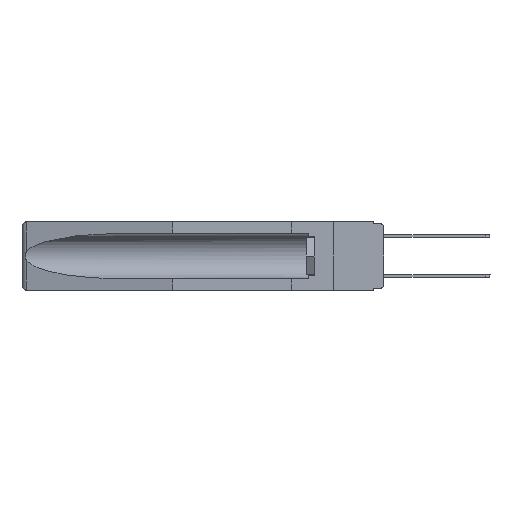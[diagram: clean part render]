
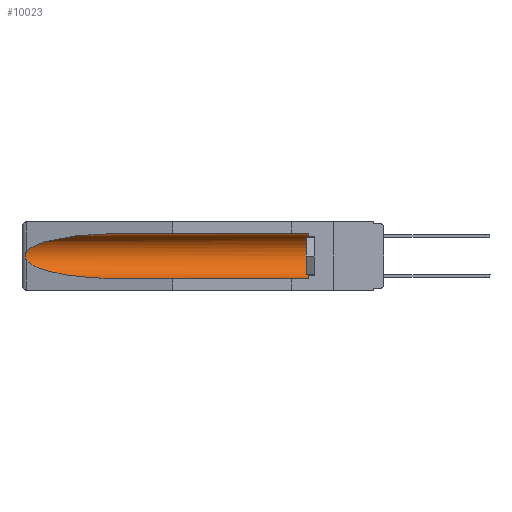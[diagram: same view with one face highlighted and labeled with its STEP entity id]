
A CAD part, left-side view. The second image highlights one B-rep face of the part: STEP entity #10023.
In plain terms, the highlighted cylindrical face has radius 2.857 mm (diameter 5.715 mm), a partial arc.
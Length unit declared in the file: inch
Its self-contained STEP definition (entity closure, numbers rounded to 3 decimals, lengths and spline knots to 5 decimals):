
#1338 = VERTEX_POINT ( 'NONE', #23030 ) ;
#1731 = CARTESIAN_POINT ( 'NONE',  ( 0.2675, 1.53308, -0.17534 ) ) ;
#1840 = CIRCLE ( 'NONE', #11067, 0.1125 ) ;
#2005 = EDGE_CURVE ( 'NONE', #6008, #21477, #17232, .T. ) ;
#2086 = CARTESIAN_POINT ( 'NONE',  ( 0.26537, 1.52718, -0.19328 ) ) ;
#2206 = CARTESIAN_POINT ( 'NONE',  ( 0.26537, 1.52718, -0.14972 ) ) ;
#2454 = EDGE_CURVE ( 'NONE', #6008, #16676, #1840, .T. ) ;
#2832 = CARTESIAN_POINT ( 'NONE',  ( 0.26537, 1.52718, -0.19328 ) ) ;
#2895 = CYLINDRICAL_SURFACE ( 'NONE', #17356, 0.1125 ) ;
#3314 = CARTESIAN_POINT ( 'NONE',  ( 0.21114, 1.30732, -0.059 ) ) ;
#3514 = EDGE_CURVE ( 'NONE', #6287, #1338, #10824, .T. ) ;
#4828 = DIRECTION ( 'NONE',  ( 0., 0., 1. ) ) ;
#5170 = CARTESIAN_POINT ( 'NONE',  ( 0.155, 0.126, -0.1715 ) ) ;
#5464 = CARTESIAN_POINT ( 'NONE',  ( 0.2673, 1.53269, -0.17917 ) ) ;
#6008 = VERTEX_POINT ( 'NONE', #12097 ) ;
#6287 = VERTEX_POINT ( 'NONE', #7847 ) ;
#6737 = DIRECTION ( 'NONE',  ( 0., 0., 1. ) ) ;
#7717 =( BOUNDED_CURVE ( )  B_SPLINE_CURVE ( 3, ( #8172, #22189, #13104, #16947 ),
 .UNSPECIFIED., .F., .T. ) 
 B_SPLINE_CURVE_WITH_KNOTS ( ( 4, 4 ),
 ( 0.1948, 1.5708 ),
 .UNSPECIFIED. ) 
 CURVE ( )  GEOMETRIC_REPRESENTATION_ITEM ( )  RATIONAL_B_SPLINE_CURVE ( ( 1., 0.848, 0.848, 1. ) ) 
 REPRESENTATION_ITEM ( '' )  );
#7847 = CARTESIAN_POINT ( 'NONE',  ( 0.155, 1.07973, -0.059 ) ) ;
#7848 = CARTESIAN_POINT ( 'NONE',  ( 0.155, -0.30754, -0.284 ) ) ;
#8172 = CARTESIAN_POINT ( 'NONE',  ( 0.26537, 1.52718, -0.19328 ) ) ;
#8545 = FACE_OUTER_BOUND ( 'NONE', #16139, .T. ) ;
#9189 = CARTESIAN_POINT ( 'NONE',  ( 0.2675, 1.53308, -0.16763 ) ) ;
#9327 = EDGE_CURVE ( 'NONE', #1338, #11338, #22212, .T. ) ;
#9767 = DIRECTION ( 'NONE',  ( 0., 1., 0. ) ) ;
#10000 = ORIENTED_EDGE ( 'NONE', *, *, #23014, .T. ) ;
#10023 = ADVANCED_FACE ( 'NONE', ( #8545 ), #2895, .F. ) ;
#10462 = ORIENTED_EDGE ( 'NONE', *, *, #3514, .T. ) ;
#10824 =( BOUNDED_CURVE ( )  B_SPLINE_CURVE ( 3, ( #23434, #3314, #16265, #23548 ),
 .UNSPECIFIED., .F., .T. ) 
 B_SPLINE_CURVE_WITH_KNOTS ( ( 4, 4 ),
 ( 4.71239, 6.08839 ),
 .UNSPECIFIED. ) 
 CURVE ( )  GEOMETRIC_REPRESENTATION_ITEM ( )  RATIONAL_B_SPLINE_CURVE ( ( 1., 0.848, 0.848, 1. ) ) 
 REPRESENTATION_ITEM ( '' )  );
#10958 = LINE ( 'NONE', #22303, #19445 ) ;
#11067 = AXIS2_PLACEMENT_3D ( 'NONE', #5170, #21582, #6737 ) ;
#11164 = CARTESIAN_POINT ( 'NONE',  ( 0.155, 1.07973, -0.284 ) ) ;
#11170 = CARTESIAN_POINT ( 'NONE',  ( 0.155, 0.126, -0.059 ) ) ;
#11338 = VERTEX_POINT ( 'NONE', #2832 ) ;
#11511 = ORIENTED_EDGE ( 'NONE', *, *, #2454, .T. ) ;
#11574 = ORIENTED_EDGE ( 'NONE', *, *, #9327, .T. ) ;
#12097 = CARTESIAN_POINT ( 'NONE',  ( 0.155, 0.126, -0.284 ) ) ;
#12155 = DIRECTION ( 'NONE',  ( 0., 1., 0. ) ) ;
#13104 = CARTESIAN_POINT ( 'NONE',  ( 0.21114, 1.30732, -0.284 ) ) ;
#13964 = ORIENTED_EDGE ( 'NONE', *, *, #16272, .T. ) ;
#14418 = VECTOR ( 'NONE', #9767, 39.37008 ) ;
#15137 = DIRECTION ( 'NONE',  ( 0., 1., 0. ) ) ;
#16139 = EDGE_LOOP ( 'NONE', ( #10462, #11574, #10000, #21799, #11511, #13964 ) ) ;
#16265 = CARTESIAN_POINT ( 'NONE',  ( 0.25451, 1.48313, -0.09465 ) ) ;
#16272 = EDGE_CURVE ( 'NONE', #16676, #6287, #10958, .T. ) ;
#16393 = CARTESIAN_POINT ( 'NONE',  ( 0.26654, 1.53092, -0.15636 ) ) ;
#16676 = VERTEX_POINT ( 'NONE', #11170 ) ;
#16748 = CARTESIAN_POINT ( 'NONE',  ( 0.26655, 1.53094, -0.18657 ) ) ;
#16947 = CARTESIAN_POINT ( 'NONE',  ( 0.155, 1.07973, -0.284 ) ) ;
#17232 = LINE ( 'NONE', #7848, #14418 ) ;
#17356 = AXIS2_PLACEMENT_3D ( 'NONE', #19577, #12155, #4828 ) ;
#19445 = VECTOR ( 'NONE', #15137, 39.37008 ) ;
#19577 = CARTESIAN_POINT ( 'NONE',  ( 0.155, -0.30754, -0.1715 ) ) ;
#20546 = CARTESIAN_POINT ( 'NONE',  ( 0.2673, 1.5327, -0.16383 ) ) ;
#21477 = VERTEX_POINT ( 'NONE', #11164 ) ;
#21582 = DIRECTION ( 'NONE',  ( 0., -1., 0. ) ) ;
#21799 = ORIENTED_EDGE ( 'NONE', *, *, #2005, .F. ) ;
#21872 = CARTESIAN_POINT ( 'NONE',  ( 0.26597, 1.52961, -0.15275 ) ) ;
#22189 = CARTESIAN_POINT ( 'NONE',  ( 0.25451, 1.48313, -0.24835 ) ) ;
#22212 = B_SPLINE_CURVE_WITH_KNOTS ( 'NONE', 3,
 ( #2206, #21872, #16393, #20546, #9189, #1731, #5464, #16748, #23675, #2086 ),
 .UNSPECIFIED., .F., .F.,
 ( 4, 2, 2, 2, 4 ),
 ( 0., 0.00029, 0.00058, 0.00087, 0.00117 ),
 .UNSPECIFIED. ) ;
#22303 = CARTESIAN_POINT ( 'NONE',  ( 0.155, -0.30754, -0.059 ) ) ;
#23014 = EDGE_CURVE ( 'NONE', #11338, #21477, #7717, .T. ) ;
#23030 = CARTESIAN_POINT ( 'NONE',  ( 0.26537, 1.52718, -0.14972 ) ) ;
#23434 = CARTESIAN_POINT ( 'NONE',  ( 0.155, 1.07973, -0.059 ) ) ;
#23548 = CARTESIAN_POINT ( 'NONE',  ( 0.26537, 1.52718, -0.14972 ) ) ;
#23675 = CARTESIAN_POINT ( 'NONE',  ( 0.26597, 1.5296, -0.19026 ) ) ;
